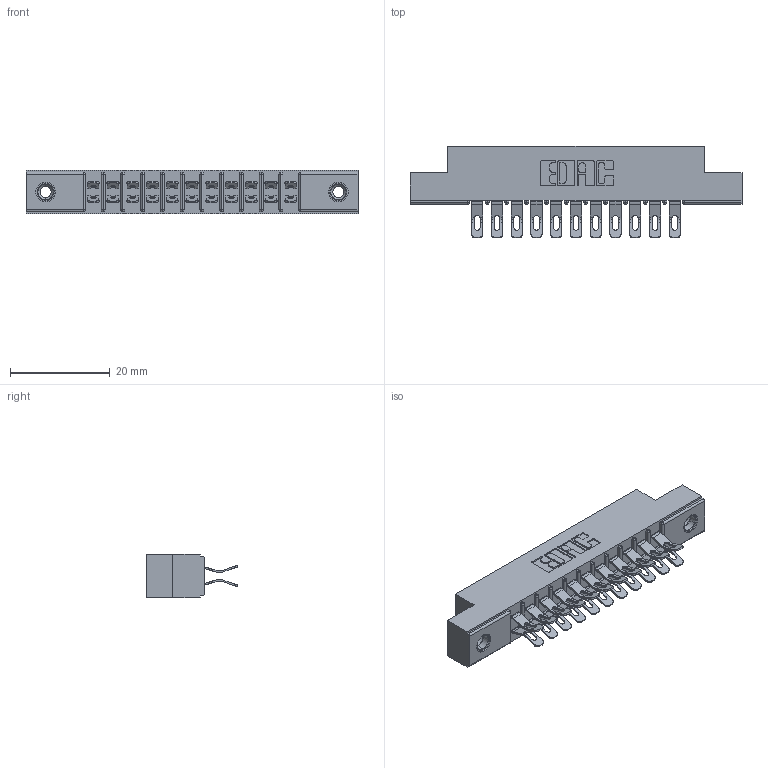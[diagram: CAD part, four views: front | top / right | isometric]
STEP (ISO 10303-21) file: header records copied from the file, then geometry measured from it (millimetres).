
FILE_DESCRIPTION (( 'STEP AP203' ), '1' );
FILE_NAME ('315-022-555-208.STEP', '2019-09-10T14:30:20', ( '' ), ( '' ), 'SwSTEP 2.0', 'SolidWorks 2016', '' );
FILE_SCHEMA (( 'CONFIG_CONTROL_DESIGN' ));
Length unit declared in the file: inch
Products named in the file (4): 305 Part_.156 Dia; 345-250-001_345-250-003-102; 305-290-001_555; 315-022-555-208
Assembly tree (25 placements, depth 2):
  315-022-555-208
    305 Part_.156 Dia
    305-290-001_555  x22
    345-250-001_345-250-003-102  x2
Bounding box: 66.6 x 18.41 x 8.71 mm (x, y, z)
Volume: 4256.1 mm3; surface area: 7774.9 mm2
Topology: 25 solids, 25 shells, 1628 faces, 4797 edges, 3130 vertices
Faces by surface type: plane 804, cylinder 764, sphere 44, cone 12, torus 4
Entity records: 17493 total; most frequent: CARTESIAN_POINT 2896, ORIENTED_EDGE 2854, DIRECTION 2831, EDGE_CURVE 1427, VECTOR 1097, LINE 1097, VERTEX_POINT 916, AXIS2_PLACEMENT_3D 867
